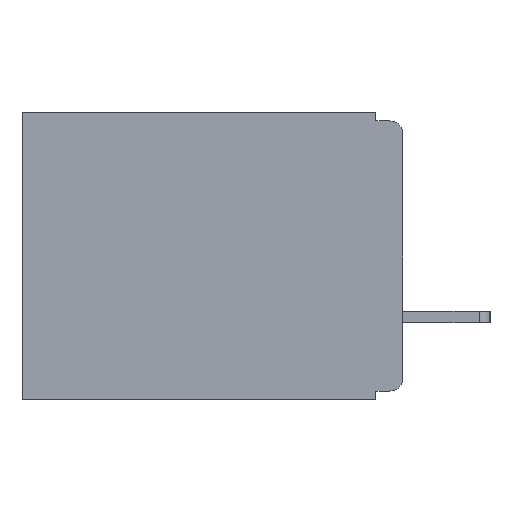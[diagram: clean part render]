
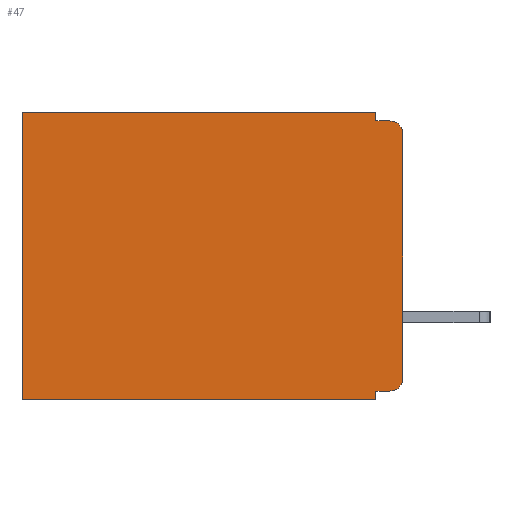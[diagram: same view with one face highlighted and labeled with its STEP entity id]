
A CAD part, left-side view. The second image highlights one B-rep face of the part: STEP entity #47.
In plain terms, the highlighted planar face has unit normal (-1, 0, 0).
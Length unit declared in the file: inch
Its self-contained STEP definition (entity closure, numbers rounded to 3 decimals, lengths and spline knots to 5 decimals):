
#47 = ADVANCED_FACE ( 'NONE', ( #16074 ), #11328, .F. ) ;
#492 = ORIENTED_EDGE ( 'NONE', *, *, #19906, .F. ) ;
#505 = CARTESIAN_POINT ( 'NONE',  ( 0.3, 0.015, -0.01 ) ) ;
#825 = LINE ( 'NONE', #19952, #19332 ) ;
#1312 = VECTOR ( 'NONE', #4730, 39.37008 ) ;
#1505 = EDGE_CURVE ( 'NONE', #14154, #19460, #6831, .T. ) ;
#1573 = CARTESIAN_POINT ( 'NONE',  ( 0.3, 0., -0.33 ) ) ;
#1612 = LINE ( 'NONE', #16392, #15473 ) ;
#1709 = VERTEX_POINT ( 'NONE', #14930 ) ;
#1827 = ORIENTED_EDGE ( 'NONE', *, *, #7394, .T. ) ;
#1959 = VECTOR ( 'NONE', #6350, 39.37008 ) ;
#2516 = CIRCLE ( 'NONE', #11524, 0.015 ) ;
#2573 = DIRECTION ( 'NONE',  ( 0., 0., -1. ) ) ;
#2885 = CIRCLE ( 'NONE', #23092, 0.015 ) ;
#3897 = VERTEX_POINT ( 'NONE', #5197 ) ;
#3913 = VERTEX_POINT ( 'NONE', #6380 ) ;
#3920 = CARTESIAN_POINT ( 'NONE',  ( 0.3, 0., -0.32 ) ) ;
#4730 = DIRECTION ( 'NONE',  ( 0., 0., -1. ) ) ;
#4815 = EDGE_LOOP ( 'NONE', ( #22751, #19570, #492, #14410, #14480, #1827, #16234, #5544, #11002, #18108 ) ) ;
#4882 = CARTESIAN_POINT ( 'NONE',  ( 0.3, 0.015, -0.305 ) ) ;
#5030 = CARTESIAN_POINT ( 'NONE',  ( 0.3, 0., -0.33 ) ) ;
#5102 = LINE ( 'NONE', #1573, #14162 ) ;
#5197 = CARTESIAN_POINT ( 'NONE',  ( 0.3, 0.031, 0. ) ) ;
#5544 = ORIENTED_EDGE ( 'NONE', *, *, #22418, .F. ) ;
#5855 = CARTESIAN_POINT ( 'NONE',  ( 0.3, 0.031, -0.32 ) ) ;
#6127 = CARTESIAN_POINT ( 'NONE',  ( 0.3, 0.015, -0.025 ) ) ;
#6350 = DIRECTION ( 'NONE',  ( 0., 1., 0. ) ) ;
#6380 = CARTESIAN_POINT ( 'NONE',  ( 0.3, 0.437, -0.33 ) ) ;
#6749 = DIRECTION ( 'NONE',  ( 0., 0., -1. ) ) ;
#6753 = CARTESIAN_POINT ( 'NONE',  ( 0.3, 0.015, -0.32 ) ) ;
#6831 = LINE ( 'NONE', #3920, #1959 ) ;
#7394 = EDGE_CURVE ( 'NONE', #15403, #3913, #825, .T. ) ;
#7468 = DIRECTION ( 'NONE',  ( 0., 1., 0. ) ) ;
#7932 = VECTOR ( 'NONE', #7468, 39.37008 ) ;
#7945 = LINE ( 'NONE', #22237, #12181 ) ;
#7983 = DIRECTION ( 'NONE',  ( 0., 0., -1. ) ) ;
#8074 = DIRECTION ( 'NONE',  ( 1., 0., 0. ) ) ;
#8110 = EDGE_CURVE ( 'NONE', #8346, #3913, #7945, .T. ) ;
#8172 = EDGE_CURVE ( 'NONE', #3897, #15354, #20343, .T. ) ;
#8264 = CARTESIAN_POINT ( 'NONE',  ( 0.3, 0.437, 0. ) ) ;
#8346 = VERTEX_POINT ( 'NONE', #17712 ) ;
#9205 = EDGE_CURVE ( 'NONE', #3897, #15403, #22453, .T. ) ;
#10666 = LINE ( 'NONE', #15192, #22860 ) ;
#11002 = ORIENTED_EDGE ( 'NONE', *, *, #1505, .F. ) ;
#11328 = PLANE ( 'NONE',  #13596 ) ;
#11524 = AXIS2_PLACEMENT_3D ( 'NONE', #6127, #18575, #7983 ) ;
#12181 = VECTOR ( 'NONE', #13616, 39.37008 ) ;
#12504 = DIRECTION ( 'NONE',  ( 0., 0., -1. ) ) ;
#12843 = CARTESIAN_POINT ( 'NONE',  ( 0.3, 0., 0. ) ) ;
#13596 = AXIS2_PLACEMENT_3D ( 'NONE', #5030, #8074, #14538 ) ;
#13616 = DIRECTION ( 'NONE',  ( 0., 1., 0. ) ) ;
#13761 = CARTESIAN_POINT ( 'NONE',  ( 0.3, 0.031, 0. ) ) ;
#13886 = VERTEX_POINT ( 'NONE', #20154 ) ;
#14154 = VERTEX_POINT ( 'NONE', #6753 ) ;
#14162 = VECTOR ( 'NONE', #12504, 39.37008 ) ;
#14410 = ORIENTED_EDGE ( 'NONE', *, *, #8172, .F. ) ;
#14480 = ORIENTED_EDGE ( 'NONE', *, *, #9205, .T. ) ;
#14538 = DIRECTION ( 'NONE',  ( 0., 0., -1. ) ) ;
#14901 = EDGE_CURVE ( 'NONE', #14154, #13886, #2885, .T. ) ;
#14930 = CARTESIAN_POINT ( 'NONE',  ( 0.3, 0., -0.025 ) ) ;
#15192 = CARTESIAN_POINT ( 'NONE',  ( 0.3, 0.031, -0.33 ) ) ;
#15354 = VERTEX_POINT ( 'NONE', #18677 ) ;
#15403 = VERTEX_POINT ( 'NONE', #8264 ) ;
#15473 = VECTOR ( 'NONE', #19852, 39.37008 ) ;
#15668 = EDGE_CURVE ( 'NONE', #1709, #13886, #5102, .T. ) ;
#16074 = FACE_OUTER_BOUND ( 'NONE', #4815, .T. ) ;
#16234 = ORIENTED_EDGE ( 'NONE', *, *, #8110, .F. ) ;
#16392 = CARTESIAN_POINT ( 'NONE',  ( 0.3, 0., -0.01 ) ) ;
#16440 = EDGE_CURVE ( 'NONE', #1709, #23090, #2516, .T. ) ;
#16560 = DIRECTION ( 'NONE',  ( 0., 0., -1. ) ) ;
#17399 = DIRECTION ( 'NONE',  ( -1., 0., 0. ) ) ;
#17712 = CARTESIAN_POINT ( 'NONE',  ( 0.3, 0.031, -0.33 ) ) ;
#18108 = ORIENTED_EDGE ( 'NONE', *, *, #14901, .T. ) ;
#18575 = DIRECTION ( 'NONE',  ( -1., 0., 0. ) ) ;
#18677 = CARTESIAN_POINT ( 'NONE',  ( 0.3, 0.031, -0.01 ) ) ;
#19332 = VECTOR ( 'NONE', #16560, 39.37008 ) ;
#19460 = VERTEX_POINT ( 'NONE', #5855 ) ;
#19570 = ORIENTED_EDGE ( 'NONE', *, *, #16440, .T. ) ;
#19852 = DIRECTION ( 'NONE',  ( 0., -1., 0. ) ) ;
#19906 = EDGE_CURVE ( 'NONE', #15354, #23090, #1612, .T. ) ;
#19952 = CARTESIAN_POINT ( 'NONE',  ( 0.3, 0.437, -0.33 ) ) ;
#20154 = CARTESIAN_POINT ( 'NONE',  ( 0.3, 0., -0.305 ) ) ;
#20343 = LINE ( 'NONE', #13761, #1312 ) ;
#22237 = CARTESIAN_POINT ( 'NONE',  ( 0.3, 0., -0.33 ) ) ;
#22418 = EDGE_CURVE ( 'NONE', #19460, #8346, #10666, .T. ) ;
#22453 = LINE ( 'NONE', #12843, #7932 ) ;
#22751 = ORIENTED_EDGE ( 'NONE', *, *, #15668, .F. ) ;
#22860 = VECTOR ( 'NONE', #2573, 39.37008 ) ;
#23090 = VERTEX_POINT ( 'NONE', #505 ) ;
#23092 = AXIS2_PLACEMENT_3D ( 'NONE', #4882, #17399, #6749 ) ;
